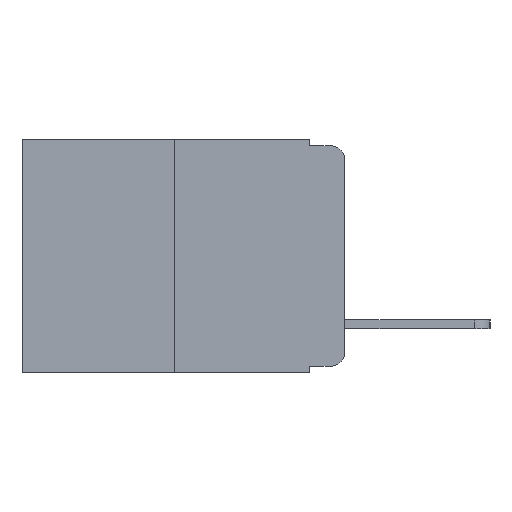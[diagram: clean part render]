
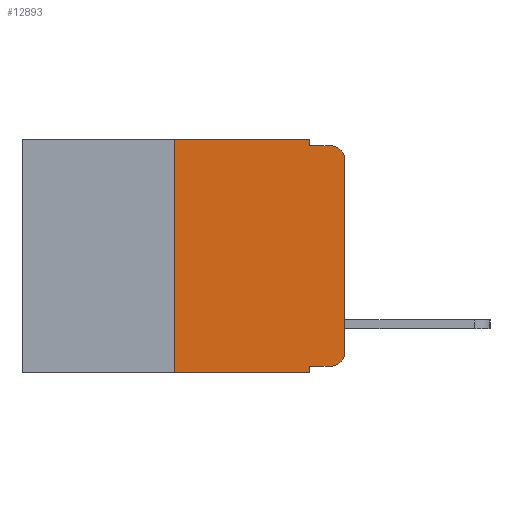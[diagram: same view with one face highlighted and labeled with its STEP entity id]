
A CAD part, left-side view. The second image highlights one B-rep face of the part: STEP entity #12893.
In plain terms, the highlighted planar face has unit normal (-1, 0, 0).
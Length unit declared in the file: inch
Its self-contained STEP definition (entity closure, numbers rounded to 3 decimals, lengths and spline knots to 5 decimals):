
#79 = DIRECTION ( 'NONE',  ( 0., 0., -1. ) ) ;
#939 = ORIENTED_EDGE ( 'NONE', *, *, #11987, .T. ) ;
#1195 = LINE ( 'NONE', #13218, #10651 ) ;
#1234 = DIRECTION ( 'NONE',  ( 0., 0., 1. ) ) ;
#1429 = ORIENTED_EDGE ( 'NONE', *, *, #10434, .F. ) ;
#1467 = VERTEX_POINT ( 'NONE', #11433 ) ;
#1518 = CARTESIAN_POINT ( 'NONE',  ( 0., 0.02, -0.313 ) ) ;
#1855 = ORIENTED_EDGE ( 'NONE', *, *, #9673, .F. ) ;
#2247 = CARTESIAN_POINT ( 'NONE',  ( 0., 0.473, 0. ) ) ;
#2249 = DIRECTION ( 'NONE',  ( 0., 0., -1. ) ) ;
#2273 = ORIENTED_EDGE ( 'NONE', *, *, #7531, .T. ) ;
#2985 = VECTOR ( 'NONE', #15619, 39.37008 ) ;
#3532 = DIRECTION ( 'NONE',  ( 0., 0., 1. ) ) ;
#3726 = DIRECTION ( 'NONE',  ( 0., -1., 0. ) ) ;
#4864 = EDGE_CURVE ( 'NONE', #11215, #1467, #14873, .T. ) ;
#4957 = VERTEX_POINT ( 'NONE', #14533 ) ;
#5098 = VECTOR ( 'NONE', #1234, 39.37008 ) ;
#5347 = LINE ( 'NONE', #9230, #11609 ) ;
#5415 = VERTEX_POINT ( 'NONE', #6171 ) ;
#5707 = EDGE_CURVE ( 'NONE', #4957, #11215, #1195, .T. ) ;
#5818 = EDGE_CURVE ( 'NONE', #13833, #5415, #9204, .T. ) ;
#5946 = AXIS2_PLACEMENT_3D ( 'NONE', #1518, #6554, #14587 ) ;
#6022 = DIRECTION ( 'NONE',  ( 0., -1., 0. ) ) ;
#6025 = CARTESIAN_POINT ( 'NONE',  ( 0., 0.25, -0.343 ) ) ;
#6040 = ORIENTED_EDGE ( 'NONE', *, *, #5707, .T. ) ;
#6171 = CARTESIAN_POINT ( 'NONE',  ( 0., 0.051, 0. ) ) ;
#6294 = LINE ( 'NONE', #8754, #12132 ) ;
#6337 = LINE ( 'NONE', #11153, #2985 ) ;
#6503 = VECTOR ( 'NONE', #2249, 39.37008 ) ;
#6554 = DIRECTION ( 'NONE',  ( -1., 0., 0. ) ) ;
#6930 = CARTESIAN_POINT ( 'NONE',  ( 0., 0., -0.03 ) ) ;
#7202 = VECTOR ( 'NONE', #3532, 39.37008 ) ;
#7531 = EDGE_CURVE ( 'NONE', #7716, #10505, #6337, .T. ) ;
#7646 = DIRECTION ( 'NONE',  ( -1., 0., 0. ) ) ;
#7716 = VERTEX_POINT ( 'NONE', #6025 ) ;
#7877 = DIRECTION ( 'NONE',  ( 1., 0., 0. ) ) ;
#8112 = EDGE_CURVE ( 'NONE', #4957, #10505, #5347, .T. ) ;
#8415 = CARTESIAN_POINT ( 'NONE',  ( 0., 0.25, 0. ) ) ;
#8754 = CARTESIAN_POINT ( 'NONE',  ( 0., 0.051, -0.01 ) ) ;
#8835 = ORIENTED_EDGE ( 'NONE', *, *, #8112, .F. ) ;
#9075 = CIRCLE ( 'NONE', #10283, 0.02 ) ;
#9204 = LINE ( 'NONE', #2247, #13294 ) ;
#9218 = FACE_OUTER_BOUND ( 'NONE', #14256, .T. ) ;
#9230 = CARTESIAN_POINT ( 'NONE',  ( 0., 0.051, 0. ) ) ;
#9382 = CARTESIAN_POINT ( 'NONE',  ( 0., 0.25, 0. ) ) ;
#9595 = VERTEX_POINT ( 'NONE', #10574 ) ;
#9599 = CARTESIAN_POINT ( 'NONE',  ( 0., 0.051, 0. ) ) ;
#9654 = CARTESIAN_POINT ( 'NONE',  ( 0., 0.051, -0.343 ) ) ;
#9673 = EDGE_CURVE ( 'NONE', #7716, #13833, #10268, .T. ) ;
#9887 = DIRECTION ( 'NONE',  ( 0., -1., 0. ) ) ;
#10155 = CARTESIAN_POINT ( 'NONE',  ( 0., 0.473, 0. ) ) ;
#10268 = LINE ( 'NONE', #8415, #7202 ) ;
#10283 = AXIS2_PLACEMENT_3D ( 'NONE', #14459, #7646, #15541 ) ;
#10434 = EDGE_CURVE ( 'NONE', #5415, #10944, #12672, .T. ) ;
#10449 = ORIENTED_EDGE ( 'NONE', *, *, #13454, .T. ) ;
#10505 = VERTEX_POINT ( 'NONE', #9654 ) ;
#10574 = CARTESIAN_POINT ( 'NONE',  ( 0., 0.02, -0.01 ) ) ;
#10651 = VECTOR ( 'NONE', #3726, 39.37008 ) ;
#10661 = CARTESIAN_POINT ( 'NONE',  ( 0., 0.051, -0.01 ) ) ;
#10944 = VERTEX_POINT ( 'NONE', #10661 ) ;
#11153 = CARTESIAN_POINT ( 'NONE',  ( 0., 0.473, -0.343 ) ) ;
#11207 = EDGE_CURVE ( 'NONE', #10944, #9595, #6294, .T. ) ;
#11215 = VERTEX_POINT ( 'NONE', #14434 ) ;
#11433 = CARTESIAN_POINT ( 'NONE',  ( 0., 0., -0.313 ) ) ;
#11609 = VECTOR ( 'NONE', #13764, 39.37008 ) ;
#11987 = EDGE_CURVE ( 'NONE', #15233, #9595, #9075, .T. ) ;
#12132 = VECTOR ( 'NONE', #9887, 39.37008 ) ;
#12249 = ORIENTED_EDGE ( 'NONE', *, *, #4864, .T. ) ;
#12672 = LINE ( 'NONE', #9599, #6503 ) ;
#12893 = ADVANCED_FACE ( 'NONE', ( #9218 ), #14680, .F. ) ;
#13218 = CARTESIAN_POINT ( 'NONE',  ( 0., 0.051, -0.333 ) ) ;
#13294 = VECTOR ( 'NONE', #6022, 39.37008 ) ;
#13454 = EDGE_CURVE ( 'NONE', #1467, #15233, #14337, .T. ) ;
#13764 = DIRECTION ( 'NONE',  ( 0., 0., -1. ) ) ;
#13789 = ORIENTED_EDGE ( 'NONE', *, *, #11207, .F. ) ;
#13833 = VERTEX_POINT ( 'NONE', #9382 ) ;
#14146 = ORIENTED_EDGE ( 'NONE', *, *, #5818, .F. ) ;
#14256 = EDGE_LOOP ( 'NONE', ( #10449, #939, #13789, #1429, #14146, #1855, #2273, #8835, #6040, #12249 ) ) ;
#14337 = LINE ( 'NONE', #15472, #5098 ) ;
#14434 = CARTESIAN_POINT ( 'NONE',  ( 0., 0.02, -0.333 ) ) ;
#14459 = CARTESIAN_POINT ( 'NONE',  ( 0., 0.02, -0.03 ) ) ;
#14533 = CARTESIAN_POINT ( 'NONE',  ( 0., 0.051, -0.333 ) ) ;
#14587 = DIRECTION ( 'NONE',  ( 0., 0., -1. ) ) ;
#14680 = PLANE ( 'NONE',  #14991 ) ;
#14873 = CIRCLE ( 'NONE', #5946, 0.02 ) ;
#14991 = AXIS2_PLACEMENT_3D ( 'NONE', #10155, #7877, #79 ) ;
#15233 = VERTEX_POINT ( 'NONE', #6930 ) ;
#15472 = CARTESIAN_POINT ( 'NONE',  ( 0., 0., 0. ) ) ;
#15541 = DIRECTION ( 'NONE',  ( 0., 0., -1. ) ) ;
#15619 = DIRECTION ( 'NONE',  ( 0., -1., 0. ) ) ;
